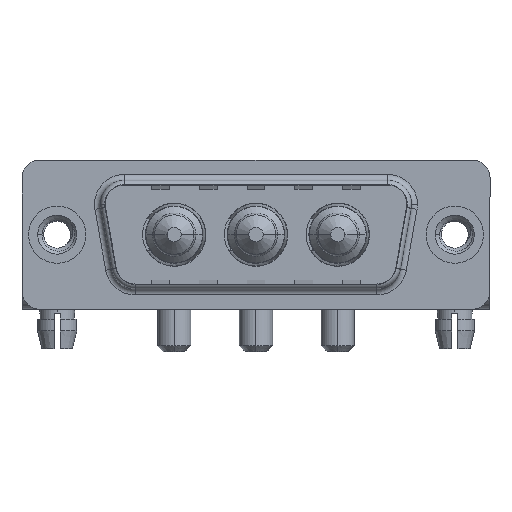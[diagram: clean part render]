
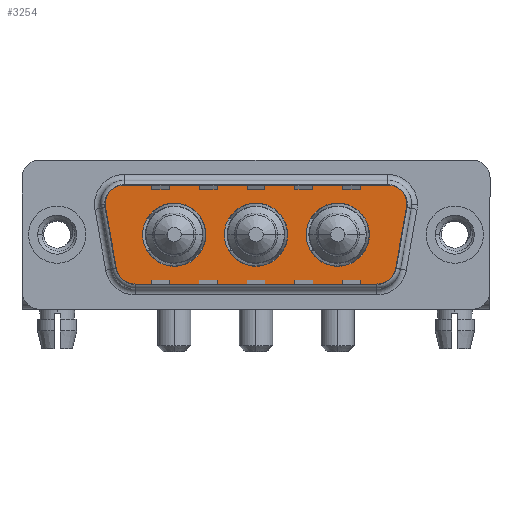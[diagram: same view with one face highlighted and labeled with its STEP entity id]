
A CAD part, top view. The second image highlights one B-rep face of the part: STEP entity #3254.
In plain terms, the highlighted planar face has unit normal (0, 0, 1).
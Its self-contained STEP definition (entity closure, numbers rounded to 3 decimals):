
#123 = EDGE_CURVE ( 'NONE', #15066, #970, #13732, .T. ) ;
#226 = VERTEX_POINT ( 'NONE', #9639 ) ;
#368 = VERTEX_POINT ( 'NONE', #13566 ) ;
#514 = EDGE_CURVE ( 'NONE', #9025, #15066, #10552, .T. ) ;
#632 = AXIS2_PLACEMENT_3D ( 'NONE', #5269, #3869, #6283 ) ;
#732 = DIRECTION ( 'NONE',  ( 0., 0., 1. ) ) ;
#743 = DIRECTION ( 'NONE',  ( 1., 0., 0. ) ) ;
#755 = ORIENTED_EDGE ( 'NONE', *, *, #14838, .F. ) ;
#772 = DIRECTION ( 'NONE',  ( -1., 0., 0. ) ) ;
#813 = AXIS2_PLACEMENT_3D ( 'NONE', #9152, #2126, #3217 ) ;
#970 = VERTEX_POINT ( 'NONE', #7195 ) ;
#1112 = CIRCLE ( 'NONE', #14604, 2. ) ;
#1373 = EDGE_LOOP ( 'NONE', ( #5099, #12612 ) ) ;
#1417 = DIRECTION ( 'NONE',  ( 1., 0., 0. ) ) ;
#1667 = EDGE_CURVE ( 'NONE', #10548, #4711, #5731, .T. ) ;
#1836 = CARTESIAN_POINT ( 'NONE',  ( 3.441, 2.553, 0. ) ) ;
#2036 = ORIENTED_EDGE ( 'NONE', *, *, #12341, .T. ) ;
#2126 = DIRECTION ( 'NONE',  ( 0., 0., 1. ) ) ;
#2293 = DIRECTION ( 'NONE',  ( 0.174, 0.985, 0. ) ) ;
#2446 = CARTESIAN_POINT ( 'NONE',  ( 29.859, 2.553, 0. ) ) ;
#2462 = EDGE_LOOP ( 'NONE', ( #755, #7540 ) ) ;
#2599 = EDGE_CURVE ( 'NONE', #14381, #9873, #8011, .T. ) ;
#2725 = FACE_BOUND ( 'NONE', #7613, .T. ) ;
#2815 = EDGE_CURVE ( 'NONE', #10495, #9537, #9006, .T. ) ;
#2945 = CARTESIAN_POINT ( 'NONE',  ( 5.411, 4.9, 0. ) ) ;
#3076 = CARTESIAN_POINT ( 'NONE',  ( 9.8, 0., 0. ) ) ;
#3212 = AXIS2_PLACEMENT_3D ( 'NONE', #13094, #4867, #14434 ) ;
#3217 = DIRECTION ( 'NONE',  ( 1., 0., 0. ) ) ;
#3254 = ADVANCED_FACE ( 'NONE', ( #2725, #13220, #13371, #8507 ), #4910, .T. ) ;
#3264 = AXIS2_PLACEMENT_3D ( 'NONE', #13021, #8602, #1417 ) ;
#3706 = DIRECTION ( 'NONE',  ( -1., 0., 0. ) ) ;
#3869 = DIRECTION ( 'NONE',  ( 0., 0., 1. ) ) ;
#3952 = EDGE_CURVE ( 'NONE', #970, #226, #8872, .T. ) ;
#3977 = DIRECTION ( 'NONE',  ( -1., 0., 0. ) ) ;
#4036 = CARTESIAN_POINT ( 'NONE',  ( 6.434, -4.9, 0. ) ) ;
#4481 = CARTESIAN_POINT ( 'NONE',  ( 20.85, 0., 0. ) ) ;
#4686 = CIRCLE ( 'NONE', #6435, 2. ) ;
#4711 = VERTEX_POINT ( 'NONE', #9015 ) ;
#4792 = CARTESIAN_POINT ( 'NONE',  ( 26.866, -2.9, 0. ) ) ;
#4833 = CARTESIAN_POINT ( 'NONE',  ( 26.866, -2.9, 0. ) ) ;
#4867 = DIRECTION ( 'NONE',  ( 0., 0., 1. ) ) ;
#4873 = CARTESIAN_POINT ( 'NONE',  ( 5.411, 4.9, 0. ) ) ;
#4910 = PLANE ( 'NONE',  #5567 ) ;
#5097 = AXIS2_PLACEMENT_3D ( 'NONE', #9001, #732, #5490 ) ;
#5099 = ORIENTED_EDGE ( 'NONE', *, *, #5748, .F. ) ;
#5269 = CARTESIAN_POINT ( 'NONE',  ( 23.5, 0., 0. ) ) ;
#5292 = DIRECTION ( 'NONE',  ( 0., 0., 1. ) ) ;
#5490 = DIRECTION ( 'NONE',  ( 1., 0., 0. ) ) ;
#5567 = AXIS2_PLACEMENT_3D ( 'NONE', #4833, #12278, #6316 ) ;
#5697 = AXIS2_PLACEMENT_3D ( 'NONE', #4792, #8536, #5805 ) ;
#5731 = LINE ( 'NONE', #2446, #10484 ) ;
#5748 = EDGE_CURVE ( 'NONE', #9873, #14381, #6599, .T. ) ;
#5805 = DIRECTION ( 'NONE',  ( 1., 0., 0. ) ) ;
#5813 = CARTESIAN_POINT ( 'NONE',  ( 28.836, -3.247, 0. ) ) ;
#6136 = ORIENTED_EDGE ( 'NONE', *, *, #8547, .T. ) ;
#6283 = DIRECTION ( 'NONE',  ( 1., 0., 0. ) ) ;
#6295 = DIRECTION ( 'NONE',  ( 1., 0., 0. ) ) ;
#6316 = DIRECTION ( 'NONE',  ( 1., 0., 0. ) ) ;
#6435 = AXIS2_PLACEMENT_3D ( 'NONE', #12515, #5292, #3977 ) ;
#6465 = ORIENTED_EDGE ( 'NONE', *, *, #3952, .T. ) ;
#6599 = CIRCLE ( 'NONE', #5097, 2.65 ) ;
#6733 = EDGE_CURVE ( 'NONE', #13267, #10651, #9119, .T. ) ;
#6735 = CARTESIAN_POINT ( 'NONE',  ( 3.441, 2.553, 0. ) ) ;
#6792 = ORIENTED_EDGE ( 'NONE', *, *, #1667, .T. ) ;
#6827 = DIRECTION ( 'NONE',  ( 0., 0., 1. ) ) ;
#7042 = VECTOR ( 'NONE', #3706, 1000. ) ;
#7163 = VERTEX_POINT ( 'NONE', #2945 ) ;
#7195 = CARTESIAN_POINT ( 'NONE',  ( 6.434, -4.9, 0. ) ) ;
#7201 = CARTESIAN_POINT ( 'NONE',  ( 12.45, 0., 0. ) ) ;
#7447 = VERTEX_POINT ( 'NONE', #10900 ) ;
#7540 = ORIENTED_EDGE ( 'NONE', *, *, #6733, .F. ) ;
#7613 = EDGE_LOOP ( 'NONE', ( #14797, #14713 ) ) ;
#7923 = ORIENTED_EDGE ( 'NONE', *, *, #123, .T. ) ;
#7926 = EDGE_CURVE ( 'NONE', #226, #10548, #12468, .T. ) ;
#8011 = CIRCLE ( 'NONE', #8513, 2.65 ) ;
#8046 = DIRECTION ( 'NONE',  ( 0., 0., 1. ) ) ;
#8319 = CARTESIAN_POINT ( 'NONE',  ( 26.15, 0., 0. ) ) ;
#8507 = FACE_OUTER_BOUND ( 'NONE', #15032, .T. ) ;
#8513 = AXIS2_PLACEMENT_3D ( 'NONE', #3076, #6827, #743 ) ;
#8536 = DIRECTION ( 'NONE',  ( 0., 0., 1. ) ) ;
#8547 = EDGE_CURVE ( 'NONE', #368, #7447, #4686, .T. ) ;
#8602 = DIRECTION ( 'NONE',  ( 0., 0., 1. ) ) ;
#8872 = LINE ( 'NONE', #4036, #12358 ) ;
#9001 = CARTESIAN_POINT ( 'NONE',  ( 9.8, 0., 0. ) ) ;
#9006 = CIRCLE ( 'NONE', #3264, 2.65 ) ;
#9015 = CARTESIAN_POINT ( 'NONE',  ( 29.859, 2.553, 0. ) ) ;
#9025 = VERTEX_POINT ( 'NONE', #1836 ) ;
#9056 = DIRECTION ( 'NONE',  ( 1., 0., 0. ) ) ;
#9119 = CIRCLE ( 'NONE', #11893, 2.65 ) ;
#9152 = CARTESIAN_POINT ( 'NONE',  ( 16.65, 0., 0. ) ) ;
#9225 = DIRECTION ( 'NONE',  ( 0.174, -0.985, 0. ) ) ;
#9355 = DIRECTION ( 'NONE',  ( 0., 0., 1. ) ) ;
#9537 = VERTEX_POINT ( 'NONE', #12311 ) ;
#9639 = CARTESIAN_POINT ( 'NONE',  ( 26.866, -4.9, 0. ) ) ;
#9723 = VECTOR ( 'NONE', #9225, 1000. ) ;
#9873 = VERTEX_POINT ( 'NONE', #7201 ) ;
#10177 = ORIENTED_EDGE ( 'NONE', *, *, #514, .T. ) ;
#10484 = VECTOR ( 'NONE', #2293, 1000. ) ;
#10495 = VERTEX_POINT ( 'NONE', #14762 ) ;
#10548 = VERTEX_POINT ( 'NONE', #5813 ) ;
#10552 = LINE ( 'NONE', #6735, #9723 ) ;
#10651 = VERTEX_POINT ( 'NONE', #8319 ) ;
#10772 = DIRECTION ( 'NONE',  ( 1., 0., 0. ) ) ;
#10790 = EDGE_CURVE ( 'NONE', #7447, #7163, #10888, .T. ) ;
#10888 = LINE ( 'NONE', #4873, #7042 ) ;
#10900 = CARTESIAN_POINT ( 'NONE',  ( 27.889, 4.9, 0. ) ) ;
#10998 = DIRECTION ( 'NONE',  ( 0., 0., 1. ) ) ;
#11067 = EDGE_CURVE ( 'NONE', #9537, #10495, #14332, .T. ) ;
#11565 = CARTESIAN_POINT ( 'NONE',  ( 5.411, 2.9, 0. ) ) ;
#11893 = AXIS2_PLACEMENT_3D ( 'NONE', #13454, #10998, #10772 ) ;
#12278 = DIRECTION ( 'NONE',  ( 0., 0., 1. ) ) ;
#12311 = CARTESIAN_POINT ( 'NONE',  ( 19.3, 0., 0. ) ) ;
#12341 = EDGE_CURVE ( 'NONE', #7163, #9025, #12399, .T. ) ;
#12358 = VECTOR ( 'NONE', #6295, 1000. ) ;
#12399 = CIRCLE ( 'NONE', #14144, 2. ) ;
#12468 = CIRCLE ( 'NONE', #5697, 2. ) ;
#12515 = CARTESIAN_POINT ( 'NONE',  ( 27.889, 2.9, 0. ) ) ;
#12612 = ORIENTED_EDGE ( 'NONE', *, *, #2599, .F. ) ;
#12749 = CARTESIAN_POINT ( 'NONE',  ( 27.889, 2.9, 0. ) ) ;
#12774 = ORIENTED_EDGE ( 'NONE', *, *, #7926, .T. ) ;
#12777 = ORIENTED_EDGE ( 'NONE', *, *, #10790, .T. ) ;
#12804 = EDGE_CURVE ( 'NONE', #4711, #368, #1112, .T. ) ;
#13021 = CARTESIAN_POINT ( 'NONE',  ( 16.65, 0., 0. ) ) ;
#13094 = CARTESIAN_POINT ( 'NONE',  ( 6.434, -2.9, 0. ) ) ;
#13128 = CIRCLE ( 'NONE', #632, 2.65 ) ;
#13220 = FACE_BOUND ( 'NONE', #2462, .T. ) ;
#13267 = VERTEX_POINT ( 'NONE', #4481 ) ;
#13371 = FACE_BOUND ( 'NONE', #1373, .T. ) ;
#13454 = CARTESIAN_POINT ( 'NONE',  ( 23.5, 0., 0. ) ) ;
#13566 = CARTESIAN_POINT ( 'NONE',  ( 29.889, 2.9, 0. ) ) ;
#13732 = CIRCLE ( 'NONE', #3212, 2. ) ;
#13891 = ORIENTED_EDGE ( 'NONE', *, *, #12804, .T. ) ;
#14144 = AXIS2_PLACEMENT_3D ( 'NONE', #11565, #8046, #9056 ) ;
#14332 = CIRCLE ( 'NONE', #813, 2.65 ) ;
#14381 = VERTEX_POINT ( 'NONE', #14769 ) ;
#14434 = DIRECTION ( 'NONE',  ( -1., 0., 0. ) ) ;
#14604 = AXIS2_PLACEMENT_3D ( 'NONE', #12749, #9355, #772 ) ;
#14713 = ORIENTED_EDGE ( 'NONE', *, *, #2815, .F. ) ;
#14762 = CARTESIAN_POINT ( 'NONE',  ( 14., 0., 0. ) ) ;
#14769 = CARTESIAN_POINT ( 'NONE',  ( 7.15, 0., 0. ) ) ;
#14797 = ORIENTED_EDGE ( 'NONE', *, *, #11067, .F. ) ;
#14838 = EDGE_CURVE ( 'NONE', #10651, #13267, #13128, .T. ) ;
#15032 = EDGE_LOOP ( 'NONE', ( #12774, #6792, #13891, #6136, #12777, #2036, #10177, #7923, #6465 ) ) ;
#15066 = VERTEX_POINT ( 'NONE', #15125 ) ;
#15125 = CARTESIAN_POINT ( 'NONE',  ( 4.464, -3.247, 0. ) ) ;
